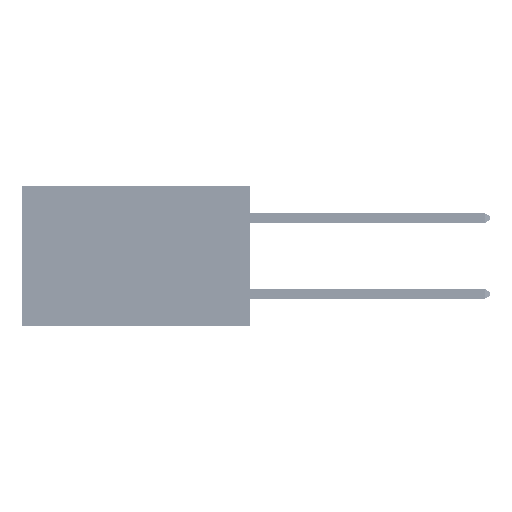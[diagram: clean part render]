
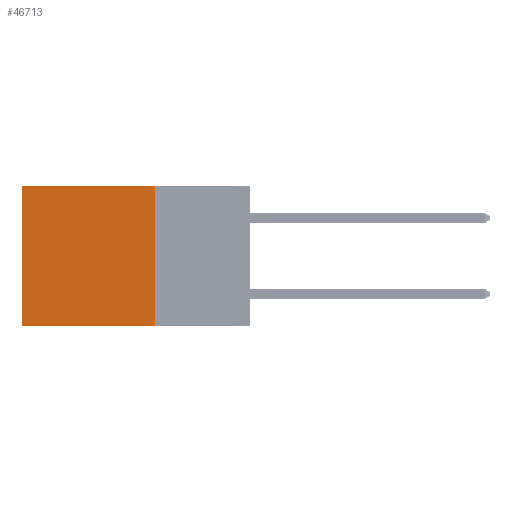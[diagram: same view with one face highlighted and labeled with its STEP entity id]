
A CAD part, left-side view. The second image highlights one B-rep face of the part: STEP entity #46713.
In plain terms, the highlighted planar face has unit normal (-1, 0, 0).
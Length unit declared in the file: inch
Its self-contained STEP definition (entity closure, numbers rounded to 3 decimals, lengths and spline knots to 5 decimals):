
#362 = VECTOR ( 'NONE', #34866, 39.37008 ) ;
#676 = EDGE_LOOP ( 'NONE', ( #22760, #19749, #12350, #23220 ) ) ;
#1037 = LINE ( 'NONE', #31062, #362 ) ;
#1975 = PLANE ( 'NONE',  #45211 ) ;
#7051 = FACE_OUTER_BOUND ( 'NONE', #676, .T. ) ;
#8785 = CARTESIAN_POINT ( 'NONE',  ( 0.2875, 0.25, 0. ) ) ;
#10614 = CARTESIAN_POINT ( 'NONE',  ( 0.2875, 0.6, 0. ) ) ;
#11470 = EDGE_CURVE ( 'NONE', #41980, #32014, #1037, .T. ) ;
#12350 = ORIENTED_EDGE ( 'NONE', *, *, #12967, .F. ) ;
#12967 = EDGE_CURVE ( 'NONE', #30919, #41980, #20857, .T. ) ;
#13451 = DIRECTION ( 'NONE',  ( 1., 0., 0. ) ) ;
#15781 = EDGE_CURVE ( 'NONE', #30919, #35836, #30030, .T. ) ;
#18141 = VECTOR ( 'NONE', #47332, 39.37008 ) ;
#19393 = CARTESIAN_POINT ( 'NONE',  ( 0.2875, 0.25, -0.37 ) ) ;
#19749 = ORIENTED_EDGE ( 'NONE', *, *, #11470, .F. ) ;
#20857 = LINE ( 'NONE', #43117, #46430 ) ;
#22760 = ORIENTED_EDGE ( 'NONE', *, *, #42704, .T. ) ;
#23220 = ORIENTED_EDGE ( 'NONE', *, *, #15781, .T. ) ;
#30030 = LINE ( 'NONE', #8785, #18141 ) ;
#30637 = DIRECTION ( 'NONE',  ( 0., 0., -1. ) ) ;
#30919 = VERTEX_POINT ( 'NONE', #48052 ) ;
#31062 = CARTESIAN_POINT ( 'NONE',  ( 0.2875, 0.25, -0.37 ) ) ;
#32014 = VERTEX_POINT ( 'NONE', #42923 ) ;
#32428 = CARTESIAN_POINT ( 'NONE',  ( 0.2875, 0.25, 0. ) ) ;
#34866 = DIRECTION ( 'NONE',  ( 0., 1., 0. ) ) ;
#35836 = VERTEX_POINT ( 'NONE', #10614 ) ;
#38250 = CARTESIAN_POINT ( 'NONE',  ( 0.2875, 0.6, 0. ) ) ;
#40039 = DIRECTION ( 'NONE',  ( 0., 0., -1. ) ) ;
#40594 = VECTOR ( 'NONE', #30637, 39.37008 ) ;
#41980 = VERTEX_POINT ( 'NONE', #19393 ) ;
#42704 = EDGE_CURVE ( 'NONE', #35836, #32014, #44764, .T. ) ;
#42923 = CARTESIAN_POINT ( 'NONE',  ( 0.2875, 0.6, -0.37 ) ) ;
#43117 = CARTESIAN_POINT ( 'NONE',  ( 0.2875, 0.25, 0. ) ) ;
#44764 = LINE ( 'NONE', #38250, #40594 ) ;
#45211 = AXIS2_PLACEMENT_3D ( 'NONE', #32428, #13451, #40039 ) ;
#46430 = VECTOR ( 'NONE', #46959, 39.37008 ) ;
#46713 = ADVANCED_FACE ( 'NONE', ( #7051 ), #1975, .F. ) ;
#46959 = DIRECTION ( 'NONE',  ( 0., 0., -1. ) ) ;
#47332 = DIRECTION ( 'NONE',  ( 0., 1., 0. ) ) ;
#48052 = CARTESIAN_POINT ( 'NONE',  ( 0.2875, 0.25, 0. ) ) ;
